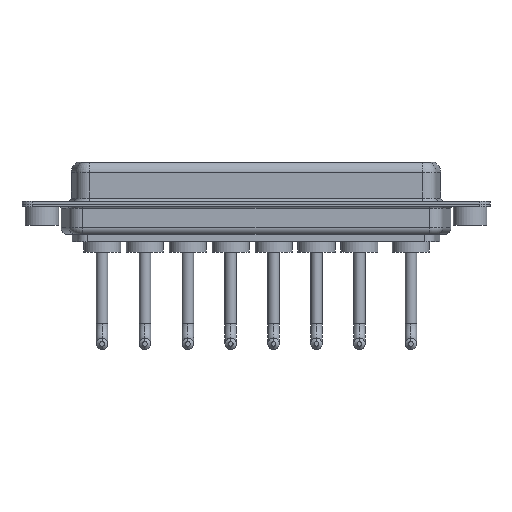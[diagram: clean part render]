
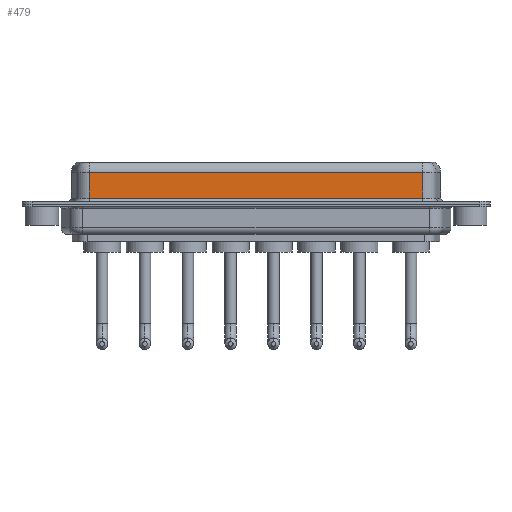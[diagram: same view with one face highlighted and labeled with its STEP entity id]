
A CAD part, front view. The second image highlights one B-rep face of the part: STEP entity #479.
In plain terms, the highlighted planar face has unit normal (0, -1, 0).
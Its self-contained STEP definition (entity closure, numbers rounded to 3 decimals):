
#85 = VECTOR ( 'NONE', #11155, 1000. ) ;
#105 = VERTEX_POINT ( 'NONE', #5291 ) ;
#479 = ADVANCED_FACE ( 'NONE', ( #12451 ), #4334, .F. ) ;
#832 = CARTESIAN_POINT ( 'NONE',  ( 56.462, -3.95, 4.65 ) ) ;
#995 = EDGE_LOOP ( 'NONE', ( #2133, #11173, #3470, #6878 ) ) ;
#1516 = EDGE_CURVE ( 'NONE', #5095, #12375, #10051, .T. ) ;
#1802 = VECTOR ( 'NONE', #7386, 1000. ) ;
#1930 = VECTOR ( 'NONE', #10614, 1000. ) ;
#2133 = ORIENTED_EDGE ( 'NONE', *, *, #1516, .F. ) ;
#2285 = CARTESIAN_POINT ( 'NONE',  ( 7.038, -3.95, 6.4 ) ) ;
#2535 = CARTESIAN_POINT ( 'NONE',  ( 7.038, -3.95, 0.9 ) ) ;
#3230 = EDGE_CURVE ( 'NONE', #105, #9476, #6523, .T. ) ;
#3470 = ORIENTED_EDGE ( 'NONE', *, *, #3230, .T. ) ;
#4149 = DIRECTION ( 'NONE',  ( 0., 0., 1. ) ) ;
#4334 = PLANE ( 'NONE',  #5281 ) ;
#4862 = LINE ( 'NONE', #832, #85 ) ;
#5095 = VERTEX_POINT ( 'NONE', #9756 ) ;
#5281 = AXIS2_PLACEMENT_3D ( 'NONE', #8429, #6402, #4149 ) ;
#5291 = CARTESIAN_POINT ( 'NONE',  ( 7.038, -3.95, 4.65 ) ) ;
#6308 = LINE ( 'NONE', #10391, #1802 ) ;
#6402 = DIRECTION ( 'NONE',  ( 0., 1., 0. ) ) ;
#6523 = LINE ( 'NONE', #2285, #1930 ) ;
#6878 = ORIENTED_EDGE ( 'NONE', *, *, #8408, .T. ) ;
#7386 = DIRECTION ( 'NONE',  ( 1., 0., 0. ) ) ;
#7906 = EDGE_CURVE ( 'NONE', #5095, #105, #4862, .T. ) ;
#8408 = EDGE_CURVE ( 'NONE', #9476, #12375, #6308, .T. ) ;
#8429 = CARTESIAN_POINT ( 'NONE',  ( 56.462, -3.95, 6.4 ) ) ;
#9293 = VECTOR ( 'NONE', #10123, 1000. ) ;
#9476 = VERTEX_POINT ( 'NONE', #2535 ) ;
#9756 = CARTESIAN_POINT ( 'NONE',  ( 56.462, -3.95, 4.65 ) ) ;
#10051 = LINE ( 'NONE', #12197, #9293 ) ;
#10123 = DIRECTION ( 'NONE',  ( 0., 0., -1. ) ) ;
#10391 = CARTESIAN_POINT ( 'NONE',  ( 56.462, -3.95, 0.9 ) ) ;
#10614 = DIRECTION ( 'NONE',  ( 0., 0., -1. ) ) ;
#11155 = DIRECTION ( 'NONE',  ( -1., 0., 0. ) ) ;
#11173 = ORIENTED_EDGE ( 'NONE', *, *, #7906, .T. ) ;
#12197 = CARTESIAN_POINT ( 'NONE',  ( 56.462, -3.95, 6.4 ) ) ;
#12375 = VERTEX_POINT ( 'NONE', #12971 ) ;
#12451 = FACE_OUTER_BOUND ( 'NONE', #995, .T. ) ;
#12971 = CARTESIAN_POINT ( 'NONE',  ( 56.462, -3.95, 0.9 ) ) ;
